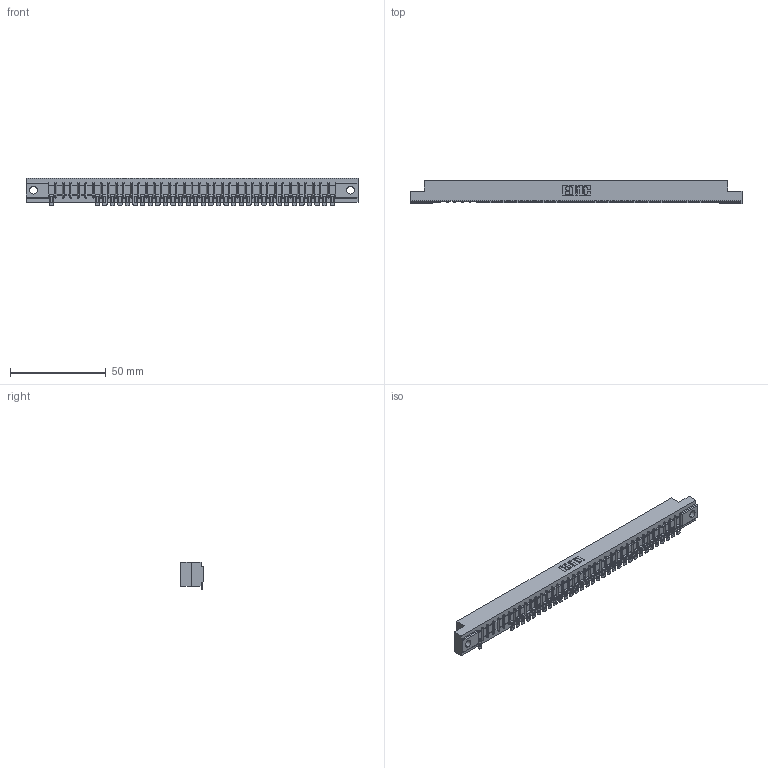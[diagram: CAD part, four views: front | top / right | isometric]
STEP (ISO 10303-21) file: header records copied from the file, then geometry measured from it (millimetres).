
FILE_DESCRIPTION (( 'STEP AP203' ), '1' );
FILE_NAME ('357-038-554-104.STEP', '2018-08-10T09:27:05', ( '' ), ( '' ), 'SwSTEP 2.0', 'SolidWorks 2016', '' );
FILE_SCHEMA (( 'CONFIG_CONTROL_DESIGN' ));
Length unit declared in the file: inch
Products named in the file (3): 307 Part_.156 Dia Mounting Holes; 307-290-002_554; 357-038-554-104
Assembly tree (34 placements, depth 2):
  357-038-554-104
    307 Part_.156 Dia Mounting Holes
    307-290-002_554  x33
Bounding box: 173.58 x 12.01 x 14.52 mm (x, y, z)
Volume: 18307.1 mm3; surface area: 21967.1 mm2
Topology: 34 solids, 34 shells, 2944 faces, 9028 edges, 5912 vertices
Faces by surface type: plane 1662, cylinder 1204, sphere 78
Entity records: 34293 total; most frequent: CARTESIAN_POINT 5811, ORIENTED_EDGE 5804, DIRECTION 5640, EDGE_CURVE 2902, VECTOR 2222, LINE 2222, VERTEX_POINT 1880, AXIS2_PLACEMENT_3D 1709
